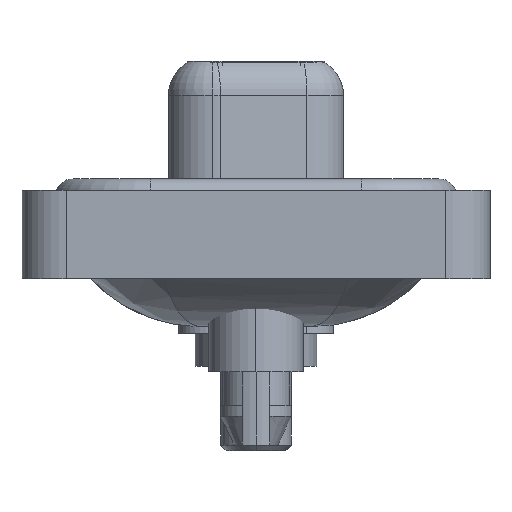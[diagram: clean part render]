
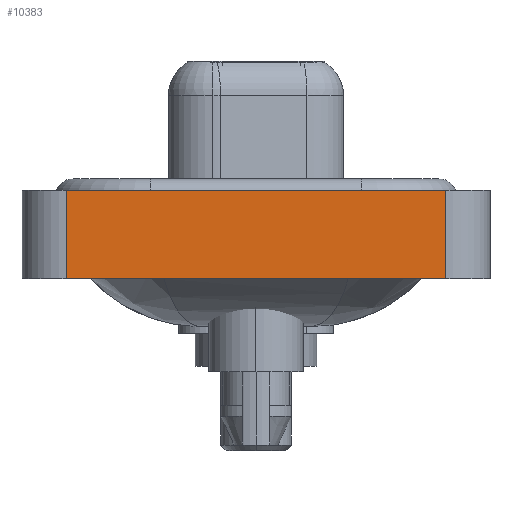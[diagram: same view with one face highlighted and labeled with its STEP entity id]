
A CAD part, left-side view. The second image highlights one B-rep face of the part: STEP entity #10383.
In plain terms, the highlighted planar face has unit normal (-1, 0, 0).
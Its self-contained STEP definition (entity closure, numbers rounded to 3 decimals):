
#568 = DIRECTION ( 'NONE',  ( 0., 0., 1. ) ) ;
#915 = DIRECTION ( 'NONE',  ( 0., -1., 0. ) ) ;
#1014 = CARTESIAN_POINT ( 'NONE',  ( -7.25, -8.55, -3.6 ) ) ;
#1367 = VECTOR ( 'NONE', #6548, 1000. ) ;
#1648 = ORIENTED_EDGE ( 'NONE', *, *, #7538, .F. ) ;
#1968 = CARTESIAN_POINT ( 'NONE',  ( -7.25, -8.55, -3.6 ) ) ;
#2203 = LINE ( 'NONE', #4888, #1367 ) ;
#2396 = PLANE ( 'NONE',  #15713 ) ;
#3681 = LINE ( 'NONE', #9321, #10123 ) ;
#4742 = FACE_OUTER_BOUND ( 'NONE', #7344, .T. ) ;
#4888 = CARTESIAN_POINT ( 'NONE',  ( -7.25, 8.55, -3.6 ) ) ;
#5149 = VERTEX_POINT ( 'NONE', #5567 ) ;
#5338 = CARTESIAN_POINT ( 'NONE',  ( -7.25, 8.55, -3.6 ) ) ;
#5479 = ORIENTED_EDGE ( 'NONE', *, *, #11725, .F. ) ;
#5567 = CARTESIAN_POINT ( 'NONE',  ( -7.25, -8.55, 0.4 ) ) ;
#5851 = ORIENTED_EDGE ( 'NONE', *, *, #8371, .T. ) ;
#6033 = CARTESIAN_POINT ( 'NONE',  ( -7.25, 8.55, 0.4 ) ) ;
#6548 = DIRECTION ( 'NONE',  ( 0., 0., 1. ) ) ;
#7344 = EDGE_LOOP ( 'NONE', ( #5851, #5479, #1648, #17508 ) ) ;
#7538 = EDGE_CURVE ( 'NONE', #10688, #10279, #2203, .T. ) ;
#8371 = EDGE_CURVE ( 'NONE', #10361, #5149, #11763, .T. ) ;
#9237 = CARTESIAN_POINT ( 'NONE',  ( -7.25, -8.55, -3.6 ) ) ;
#9321 = CARTESIAN_POINT ( 'NONE',  ( -7.25, -8.55, -3.6 ) ) ;
#10123 = VECTOR ( 'NONE', #915, 1000. ) ;
#10279 = VERTEX_POINT ( 'NONE', #6033 ) ;
#10361 = VERTEX_POINT ( 'NONE', #1014 ) ;
#10373 = DIRECTION ( 'NONE',  ( -1., 0., 0. ) ) ;
#10383 = ADVANCED_FACE ( 'NONE', ( #4742 ), #2396, .T. ) ;
#10688 = VERTEX_POINT ( 'NONE', #5338 ) ;
#11725 = EDGE_CURVE ( 'NONE', #10279, #5149, #13996, .T. ) ;
#11763 = LINE ( 'NONE', #1968, #13441 ) ;
#13441 = VECTOR ( 'NONE', #568, 1000. ) ;
#13798 = VECTOR ( 'NONE', #15216, 1000. ) ;
#13996 = LINE ( 'NONE', #18107, #13798 ) ;
#15206 = EDGE_CURVE ( 'NONE', #10688, #10361, #3681, .T. ) ;
#15216 = DIRECTION ( 'NONE',  ( 0., -1., 0. ) ) ;
#15713 = AXIS2_PLACEMENT_3D ( 'NONE', #9237, #10373, #16306 ) ;
#16306 = DIRECTION ( 'NONE',  ( 0., 0., 1. ) ) ;
#17508 = ORIENTED_EDGE ( 'NONE', *, *, #15206, .T. ) ;
#18107 = CARTESIAN_POINT ( 'NONE',  ( -7.25, -8.55, 0.4 ) ) ;
